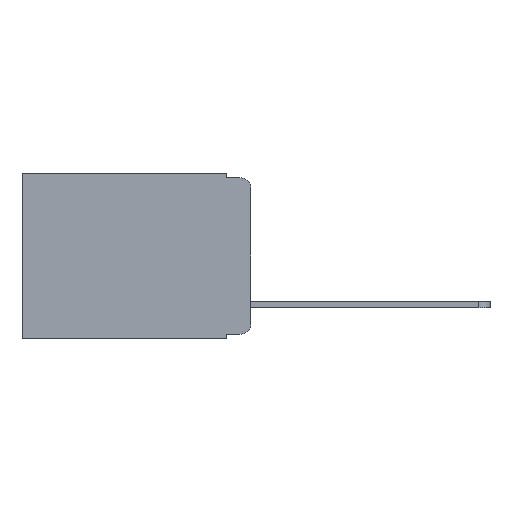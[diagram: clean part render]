
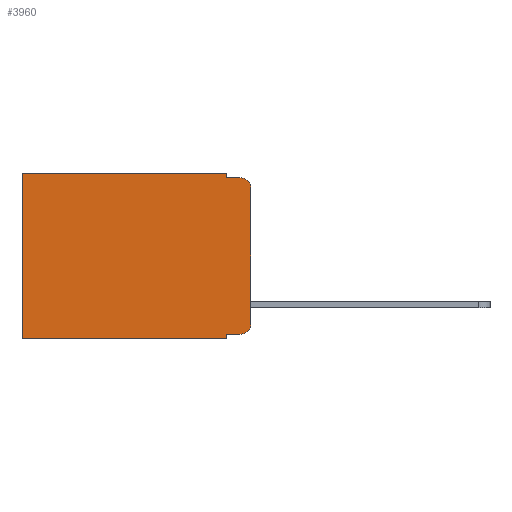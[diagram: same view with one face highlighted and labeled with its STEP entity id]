
A CAD part, left-side view. The second image highlights one B-rep face of the part: STEP entity #3960.
In plain terms, the highlighted planar face has unit normal (-1, 0, 0).
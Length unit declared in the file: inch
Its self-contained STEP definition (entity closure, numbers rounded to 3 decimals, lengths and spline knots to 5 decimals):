
#83 = DIRECTION ( 'NONE',  ( 0., 0., -1. ) ) ;
#289 = LINE ( 'NONE', #4576, #5903 ) ;
#355 = VECTOR ( 'NONE', #1912, 39.37008 ) ;
#561 = DIRECTION ( 'NONE',  ( 0., 0., -1. ) ) ;
#692 = EDGE_CURVE ( 'NONE', #8819, #4315, #3923, .T. ) ;
#787 = EDGE_CURVE ( 'NONE', #11512, #4417, #3613, .T. ) ;
#866 = DIRECTION ( 'NONE',  ( 0., 0., -1. ) ) ;
#1115 = CARTESIAN_POINT ( 'NONE',  ( 0.298, 0.02, -0.313 ) ) ;
#1139 = LINE ( 'NONE', #7824, #355 ) ;
#1912 = DIRECTION ( 'NONE',  ( 0., 1., 0. ) ) ;
#2166 = EDGE_CURVE ( 'NONE', #4315, #8696, #9669, .T. ) ;
#2337 = VECTOR ( 'NONE', #3464, 39.37008 ) ;
#2593 = ORIENTED_EDGE ( 'NONE', *, *, #692, .F. ) ;
#2679 = VECTOR ( 'NONE', #83, 39.37008 ) ;
#2966 = CARTESIAN_POINT ( 'NONE',  ( 0.298, 0.051, 0. ) ) ;
#3090 = LINE ( 'NONE', #6986, #8725 ) ;
#3325 = CARTESIAN_POINT ( 'NONE',  ( 0.298, 0.02, -0.03 ) ) ;
#3431 = DIRECTION ( 'NONE',  ( 0., 1., 0. ) ) ;
#3464 = DIRECTION ( 'NONE',  ( 0., -1., 0. ) ) ;
#3527 = ORIENTED_EDGE ( 'NONE', *, *, #2166, .F. ) ;
#3613 = LINE ( 'NONE', #10405, #12841 ) ;
#3619 = LINE ( 'NONE', #4483, #9576 ) ;
#3923 = LINE ( 'NONE', #8042, #2679 ) ;
#3960 = ADVANCED_FACE ( 'NONE', ( #4790 ), #5166, .F. ) ;
#3995 = AXIS2_PLACEMENT_3D ( 'NONE', #4248, #4338, #11267 ) ;
#4017 = CARTESIAN_POINT ( 'NONE',  ( 0.298, 0.051, -0.01 ) ) ;
#4248 = CARTESIAN_POINT ( 'NONE',  ( 0.298, 0., 0. ) ) ;
#4315 = VERTEX_POINT ( 'NONE', #4017 ) ;
#4336 = CARTESIAN_POINT ( 'NONE',  ( 0.298, 0., -0.313 ) ) ;
#4338 = DIRECTION ( 'NONE',  ( 1., 0., 0. ) ) ;
#4417 = VERTEX_POINT ( 'NONE', #12197 ) ;
#4483 = CARTESIAN_POINT ( 'NONE',  ( 0.298, 0., -0.343 ) ) ;
#4562 = CARTESIAN_POINT ( 'NONE',  ( 0.298, 0.02, -0.333 ) ) ;
#4576 = CARTESIAN_POINT ( 'NONE',  ( 0.298, 0.051, -0.333 ) ) ;
#4598 = LINE ( 'NONE', #6268, #6941 ) ;
#4648 = ORIENTED_EDGE ( 'NONE', *, *, #787, .F. ) ;
#4687 = EDGE_CURVE ( 'NONE', #7422, #10610, #3090, .T. ) ;
#4790 = FACE_OUTER_BOUND ( 'NONE', #7403, .T. ) ;
#4791 = DIRECTION ( 'NONE',  ( 0., -1., 0. ) ) ;
#4956 = ORIENTED_EDGE ( 'NONE', *, *, #6113, .T. ) ;
#5166 = PLANE ( 'NONE',  #3995 ) ;
#5505 = ORIENTED_EDGE ( 'NONE', *, *, #12278, .T. ) ;
#5675 = CARTESIAN_POINT ( 'NONE',  ( 0.298, 0.02, -0.01 ) ) ;
#5903 = VECTOR ( 'NONE', #4791, 39.37008 ) ;
#6057 = CARTESIAN_POINT ( 'NONE',  ( 0.298, 0.473, 0. ) ) ;
#6113 = EDGE_CURVE ( 'NONE', #7915, #9624, #4598, .T. ) ;
#6268 = CARTESIAN_POINT ( 'NONE',  ( 0.298, 0.473, 0. ) ) ;
#6403 = CARTESIAN_POINT ( 'NONE',  ( 0.298, 0.473, -0.343 ) ) ;
#6417 = VERTEX_POINT ( 'NONE', #4562 ) ;
#6509 = ORIENTED_EDGE ( 'NONE', *, *, #10357, .T. ) ;
#6676 = EDGE_CURVE ( 'NONE', #6417, #10610, #11136, .T. ) ;
#6856 = ORIENTED_EDGE ( 'NONE', *, *, #4687, .F. ) ;
#6941 = VECTOR ( 'NONE', #7151, 39.37008 ) ;
#6986 = CARTESIAN_POINT ( 'NONE',  ( 0.298, 0., 0. ) ) ;
#7037 = AXIS2_PLACEMENT_3D ( 'NONE', #1115, #11960, #12094 ) ;
#7151 = DIRECTION ( 'NONE',  ( 0., 0., -1. ) ) ;
#7403 = EDGE_LOOP ( 'NONE', ( #6856, #5505, #3527, #2593, #6509, #4956, #9588, #4648, #9271, #12679 ) ) ;
#7422 = VERTEX_POINT ( 'NONE', #11052 ) ;
#7824 = CARTESIAN_POINT ( 'NONE',  ( 0.298, 0., 0. ) ) ;
#7915 = VERTEX_POINT ( 'NONE', #6057 ) ;
#8042 = CARTESIAN_POINT ( 'NONE',  ( 0.298, 0.051, 0. ) ) ;
#8349 = CARTESIAN_POINT ( 'NONE',  ( 0.298, 0.051, -0.01 ) ) ;
#8696 = VERTEX_POINT ( 'NONE', #5675 ) ;
#8725 = VECTOR ( 'NONE', #866, 39.37008 ) ;
#8819 = VERTEX_POINT ( 'NONE', #2966 ) ;
#8955 = CARTESIAN_POINT ( 'NONE',  ( 0.298, 0.051, -0.333 ) ) ;
#9154 = DIRECTION ( 'NONE',  ( 0., 0., -1. ) ) ;
#9271 = ORIENTED_EDGE ( 'NONE', *, *, #12712, .T. ) ;
#9576 = VECTOR ( 'NONE', #3431, 39.37008 ) ;
#9588 = ORIENTED_EDGE ( 'NONE', *, *, #9641, .F. ) ;
#9624 = VERTEX_POINT ( 'NONE', #6403 ) ;
#9641 = EDGE_CURVE ( 'NONE', #4417, #9624, #3619, .T. ) ;
#9669 = LINE ( 'NONE', #8349, #2337 ) ;
#10090 = AXIS2_PLACEMENT_3D ( 'NONE', #3325, #12250, #9154 ) ;
#10357 = EDGE_CURVE ( 'NONE', #8819, #7915, #1139, .T. ) ;
#10405 = CARTESIAN_POINT ( 'NONE',  ( 0.298, 0.051, 0. ) ) ;
#10610 = VERTEX_POINT ( 'NONE', #4336 ) ;
#11052 = CARTESIAN_POINT ( 'NONE',  ( 0.298, 0., -0.03 ) ) ;
#11136 = CIRCLE ( 'NONE', #7037, 0.02 ) ;
#11267 = DIRECTION ( 'NONE',  ( 0., 0., -1. ) ) ;
#11512 = VERTEX_POINT ( 'NONE', #8955 ) ;
#11960 = DIRECTION ( 'NONE',  ( -1., 0., 0. ) ) ;
#12094 = DIRECTION ( 'NONE',  ( 0., 0., -1. ) ) ;
#12197 = CARTESIAN_POINT ( 'NONE',  ( 0.298, 0.051, -0.343 ) ) ;
#12250 = DIRECTION ( 'NONE',  ( -1., 0., 0. ) ) ;
#12278 = EDGE_CURVE ( 'NONE', #7422, #8696, #12463, .T. ) ;
#12463 = CIRCLE ( 'NONE', #10090, 0.02 ) ;
#12679 = ORIENTED_EDGE ( 'NONE', *, *, #6676, .T. ) ;
#12712 = EDGE_CURVE ( 'NONE', #11512, #6417, #289, .T. ) ;
#12841 = VECTOR ( 'NONE', #561, 39.37008 ) ;
